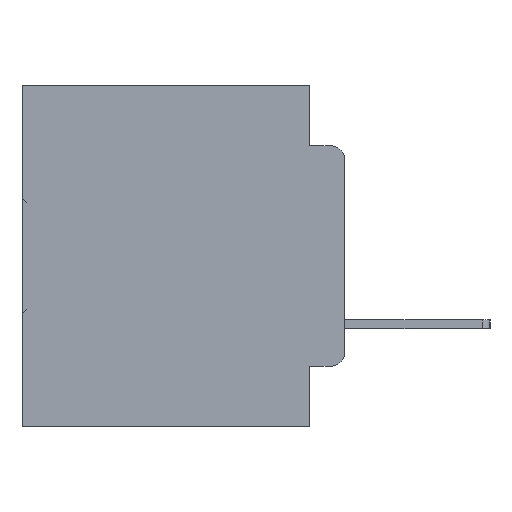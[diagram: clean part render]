
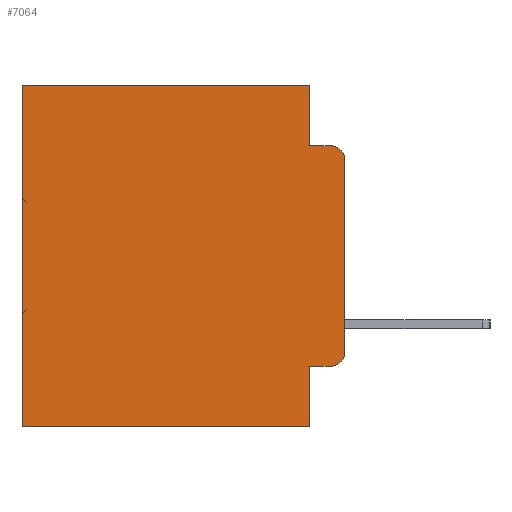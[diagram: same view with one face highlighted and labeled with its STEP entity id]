
A CAD part, left-side view. The second image highlights one B-rep face of the part: STEP entity #7064.
In plain terms, the highlighted planar face has unit normal (-1, 0, 0).
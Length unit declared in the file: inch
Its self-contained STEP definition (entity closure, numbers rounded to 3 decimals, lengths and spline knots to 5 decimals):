
#1177 = LINE ( 'NONE', #5749, #21959 ) ;
#1781 = VECTOR ( 'NONE', #29497, 39.37008 ) ;
#2856 = CARTESIAN_POINT ( 'NONE',  ( 0.298, 0.02, -0.0885 ) ) ;
#2974 = DIRECTION ( 'NONE',  ( 0., 1., 0. ) ) ;
#3051 = CARTESIAN_POINT ( 'NONE',  ( 0.298, 0.051, -0.4115 ) ) ;
#3482 = LINE ( 'NONE', #7687, #5193 ) ;
#4387 = CARTESIAN_POINT ( 'NONE',  ( 0.298, 0.051, -0.0885 ) ) ;
#5048 = EDGE_CURVE ( 'NONE', #33759, #18656, #1177, .T. ) ;
#5193 = VECTOR ( 'NONE', #31720, 39.37008 ) ;
#5280 = DIRECTION ( 'NONE',  ( -1., 0., 0. ) ) ;
#5367 = ORIENTED_EDGE ( 'NONE', *, *, #7372, .T. ) ;
#5385 = CARTESIAN_POINT ( 'NONE',  ( 0.298, 0.473, 0. ) ) ;
#5513 = CARTESIAN_POINT ( 'NONE',  ( 0.298, 0., -0.3915 ) ) ;
#5695 = CARTESIAN_POINT ( 'NONE',  ( 0.298, 0.02, -0.4115 ) ) ;
#5749 = CARTESIAN_POINT ( 'NONE',  ( 0.298, 0., -0.5 ) ) ;
#6119 = DIRECTION ( 'NONE',  ( 0., 0., -1. ) ) ;
#6175 = CARTESIAN_POINT ( 'NONE',  ( 0.298, 0.051, 0. ) ) ;
#6752 = VECTOR ( 'NONE', #8464, 39.37008 ) ;
#7064 = ADVANCED_FACE ( 'NONE', ( #15049 ), #12376, .F. ) ;
#7372 = EDGE_CURVE ( 'NONE', #33399, #8037, #20068, .T. ) ;
#7687 = CARTESIAN_POINT ( 'NONE',  ( 0.298, 0.051, -0.0885 ) ) ;
#7801 = DIRECTION ( 'NONE',  ( 0., 0., -1. ) ) ;
#7913 = ORIENTED_EDGE ( 'NONE', *, *, #33281, .F. ) ;
#8037 = VERTEX_POINT ( 'NONE', #5385 ) ;
#8055 = VERTEX_POINT ( 'NONE', #2856 ) ;
#8189 = DIRECTION ( 'NONE',  ( 0., 1., 0. ) ) ;
#8216 = LINE ( 'NONE', #10824, #1781 ) ;
#8316 = EDGE_LOOP ( 'NONE', ( #7913, #13041, #32143, #31332, #5367, #21860, #27249, #15557, #18496, #31749 ) ) ;
#8464 = DIRECTION ( 'NONE',  ( 0., 0., -1. ) ) ;
#9637 = VECTOR ( 'NONE', #11302, 39.37008 ) ;
#9752 = LINE ( 'NONE', #17016, #16091 ) ;
#9914 = AXIS2_PLACEMENT_3D ( 'NONE', #23066, #30977, #15083 ) ;
#10069 = EDGE_CURVE ( 'NONE', #21726, #22858, #18622, .T. ) ;
#10516 = CARTESIAN_POINT ( 'NONE',  ( 0.298, 0.051, 0. ) ) ;
#10824 = CARTESIAN_POINT ( 'NONE',  ( 0.298, 0.051, 0. ) ) ;
#11302 = DIRECTION ( 'NONE',  ( 0., -1., 0. ) ) ;
#11903 = EDGE_CURVE ( 'NONE', #24779, #21726, #23943, .T. ) ;
#12357 = CARTESIAN_POINT ( 'NONE',  ( 0.298, 0.473, -0.5 ) ) ;
#12376 = PLANE ( 'NONE',  #9914 ) ;
#12924 = VECTOR ( 'NONE', #8189, 39.37008 ) ;
#13041 = ORIENTED_EDGE ( 'NONE', *, *, #28047, .T. ) ;
#13712 = EDGE_CURVE ( 'NONE', #24779, #33759, #8216, .T. ) ;
#13973 = LINE ( 'NONE', #19192, #6752 ) ;
#14523 = DIRECTION ( 'NONE',  ( -1., 0., 0. ) ) ;
#15049 = FACE_OUTER_BOUND ( 'NONE', #8316, .T. ) ;
#15083 = DIRECTION ( 'NONE',  ( 0., 0., -1. ) ) ;
#15557 = ORIENTED_EDGE ( 'NONE', *, *, #13712, .F. ) ;
#15936 = CIRCLE ( 'NONE', #21215, 0.02 ) ;
#16091 = VECTOR ( 'NONE', #6119, 39.37008 ) ;
#16219 = CARTESIAN_POINT ( 'NONE',  ( 0.298, 0., 0. ) ) ;
#17016 = CARTESIAN_POINT ( 'NONE',  ( 0.298, 0.473, 0. ) ) ;
#18496 = ORIENTED_EDGE ( 'NONE', *, *, #11903, .T. ) ;
#18622 = CIRCLE ( 'NONE', #21268, 0.02 ) ;
#18656 = VERTEX_POINT ( 'NONE', #12357 ) ;
#18747 = VERTEX_POINT ( 'NONE', #31407 ) ;
#19105 = EDGE_CURVE ( 'NONE', #8037, #18656, #9752, .T. ) ;
#19192 = CARTESIAN_POINT ( 'NONE',  ( 0.298, 0., 0. ) ) ;
#19746 = VECTOR ( 'NONE', #7801, 39.37008 ) ;
#20068 = LINE ( 'NONE', #16219, #12924 ) ;
#20909 = EDGE_CURVE ( 'NONE', #33399, #26402, #34578, .T. ) ;
#21215 = AXIS2_PLACEMENT_3D ( 'NONE', #30437, #14523, #33070 ) ;
#21268 = AXIS2_PLACEMENT_3D ( 'NONE', #21489, #5280, #24150 ) ;
#21456 = CARTESIAN_POINT ( 'NONE',  ( 0.298, 0.051, -0.4115 ) ) ;
#21489 = CARTESIAN_POINT ( 'NONE',  ( 0.298, 0.02, -0.3915 ) ) ;
#21726 = VERTEX_POINT ( 'NONE', #5695 ) ;
#21860 = ORIENTED_EDGE ( 'NONE', *, *, #19105, .T. ) ;
#21959 = VECTOR ( 'NONE', #2974, 39.37008 ) ;
#22729 = EDGE_CURVE ( 'NONE', #26402, #8055, #3482, .T. ) ;
#22858 = VERTEX_POINT ( 'NONE', #5513 ) ;
#23066 = CARTESIAN_POINT ( 'NONE',  ( 0.298, 0., 0. ) ) ;
#23943 = LINE ( 'NONE', #3051, #9637 ) ;
#24150 = DIRECTION ( 'NONE',  ( 0., 0., -1. ) ) ;
#24779 = VERTEX_POINT ( 'NONE', #21456 ) ;
#26402 = VERTEX_POINT ( 'NONE', #4387 ) ;
#27249 = ORIENTED_EDGE ( 'NONE', *, *, #5048, .F. ) ;
#28047 = EDGE_CURVE ( 'NONE', #18747, #8055, #15936, .T. ) ;
#29497 = DIRECTION ( 'NONE',  ( 0., 0., -1. ) ) ;
#30437 = CARTESIAN_POINT ( 'NONE',  ( 0.298, 0.02, -0.1085 ) ) ;
#30977 = DIRECTION ( 'NONE',  ( 1., 0., 0. ) ) ;
#31332 = ORIENTED_EDGE ( 'NONE', *, *, #20909, .F. ) ;
#31407 = CARTESIAN_POINT ( 'NONE',  ( 0.298, 0., -0.1085 ) ) ;
#31720 = DIRECTION ( 'NONE',  ( 0., -1., 0. ) ) ;
#31744 = CARTESIAN_POINT ( 'NONE',  ( 0.298, 0.051, -0.5 ) ) ;
#31749 = ORIENTED_EDGE ( 'NONE', *, *, #10069, .T. ) ;
#32143 = ORIENTED_EDGE ( 'NONE', *, *, #22729, .F. ) ;
#33070 = DIRECTION ( 'NONE',  ( 0., 0., -1. ) ) ;
#33281 = EDGE_CURVE ( 'NONE', #18747, #22858, #13973, .T. ) ;
#33399 = VERTEX_POINT ( 'NONE', #6175 ) ;
#33759 = VERTEX_POINT ( 'NONE', #31744 ) ;
#34578 = LINE ( 'NONE', #10516, #19746 ) ;
